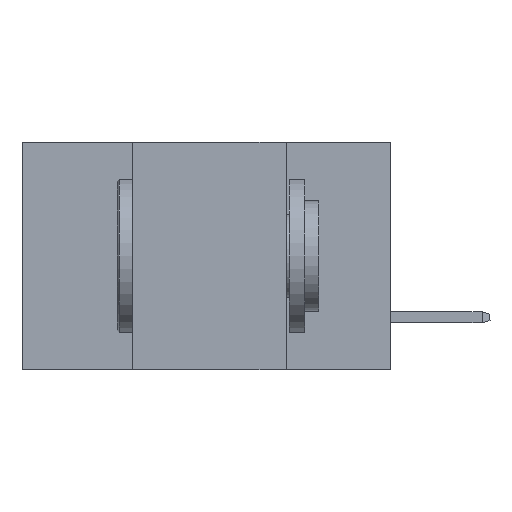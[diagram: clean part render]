
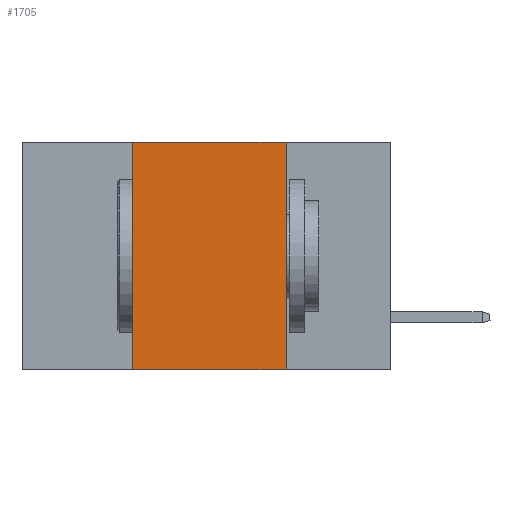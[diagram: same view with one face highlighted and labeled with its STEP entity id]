
A CAD part, left-side view. The second image highlights one B-rep face of the part: STEP entity #1705.
In plain terms, the highlighted planar face has unit normal (-1, 0, 0).
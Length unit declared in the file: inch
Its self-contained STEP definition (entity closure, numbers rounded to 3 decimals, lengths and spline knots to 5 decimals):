
#682 = VERTEX_POINT ( 'NONE', #2713 ) ;
#945 = VECTOR ( 'NONE', #1400, 39.37008 ) ;
#1362 = CARTESIAN_POINT ( 'NONE',  ( 0., 0.6, 0. ) ) ;
#1400 = DIRECTION ( 'NONE',  ( 0., -1., 0. ) ) ;
#1527 = DIRECTION ( 'NONE',  ( 0., -1., 0. ) ) ;
#1648 = CARTESIAN_POINT ( 'NONE',  ( 0., 0.6, 0. ) ) ;
#1705 = ADVANCED_FACE ( 'NONE', ( #3393 ), #1816, .F. ) ;
#1816 = PLANE ( 'NONE',  #5487 ) ;
#1994 = VERTEX_POINT ( 'NONE', #5612 ) ;
#1996 = LINE ( 'NONE', #1362, #5772 ) ;
#2100 = VERTEX_POINT ( 'NONE', #3180 ) ;
#2498 = EDGE_LOOP ( 'NONE', ( #5637, #3206, #3096, #3671 ) ) ;
#2581 = DIRECTION ( 'NONE',  ( 0., 0., -1. ) ) ;
#2713 = CARTESIAN_POINT ( 'NONE',  ( 0., 0.42, 0. ) ) ;
#3096 = ORIENTED_EDGE ( 'NONE', *, *, #8519, .F. ) ;
#3180 = CARTESIAN_POINT ( 'NONE',  ( 0., 0.42, -0.37 ) ) ;
#3206 = ORIENTED_EDGE ( 'NONE', *, *, #4570, .F. ) ;
#3393 = FACE_OUTER_BOUND ( 'NONE', #2498, .T. ) ;
#3579 = DIRECTION ( 'NONE',  ( 1., 0., 0. ) ) ;
#3671 = ORIENTED_EDGE ( 'NONE', *, *, #10363, .T. ) ;
#4026 = VECTOR ( 'NONE', #8647, 39.37008 ) ;
#4331 = LINE ( 'NONE', #10154, #6620 ) ;
#4570 = EDGE_CURVE ( 'NONE', #682, #10472, #1996, .T. ) ;
#5440 = DIRECTION ( 'NONE',  ( 0., 0., 1. ) ) ;
#5487 = AXIS2_PLACEMENT_3D ( 'NONE', #1648, #3579, #2581 ) ;
#5612 = CARTESIAN_POINT ( 'NONE',  ( 0., 0.17, -0.37 ) ) ;
#5637 = ORIENTED_EDGE ( 'NONE', *, *, #10129, .F. ) ;
#5772 = VECTOR ( 'NONE', #1527, 39.37008 ) ;
#6057 = CARTESIAN_POINT ( 'NONE',  ( 0., 0.17, 0. ) ) ;
#6205 = LINE ( 'NONE', #8979, #945 ) ;
#6620 = VECTOR ( 'NONE', #5440, 39.37008 ) ;
#8228 = LINE ( 'NONE', #9414, #4026 ) ;
#8519 = EDGE_CURVE ( 'NONE', #2100, #682, #4331, .T. ) ;
#8647 = DIRECTION ( 'NONE',  ( 0., 0., -1. ) ) ;
#8979 = CARTESIAN_POINT ( 'NONE',  ( 0., 0.6, -0.37 ) ) ;
#9414 = CARTESIAN_POINT ( 'NONE',  ( 0., 0.17, 0. ) ) ;
#10129 = EDGE_CURVE ( 'NONE', #10472, #1994, #8228, .T. ) ;
#10154 = CARTESIAN_POINT ( 'NONE',  ( 0., 0.42, 0. ) ) ;
#10363 = EDGE_CURVE ( 'NONE', #2100, #1994, #6205, .T. ) ;
#10472 = VERTEX_POINT ( 'NONE', #6057 ) ;
